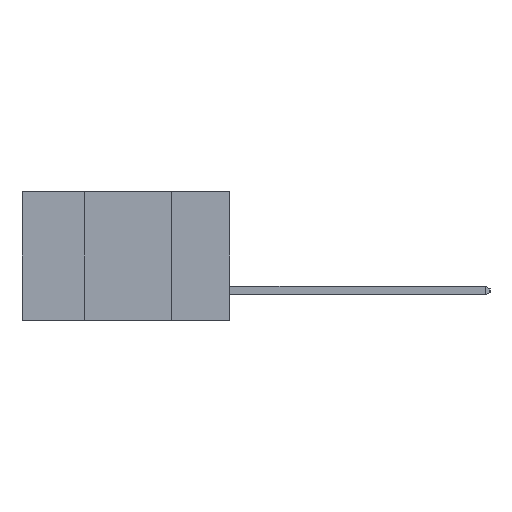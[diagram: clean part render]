
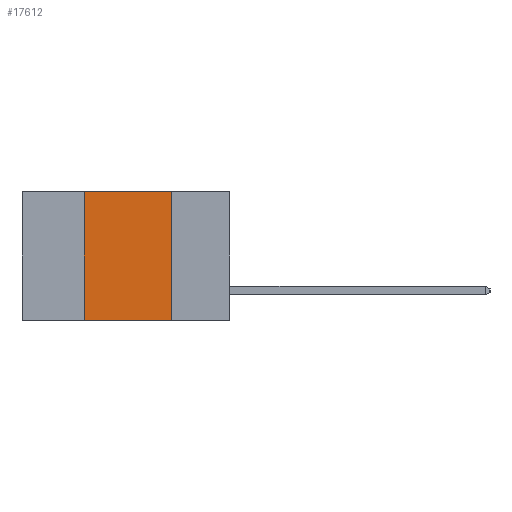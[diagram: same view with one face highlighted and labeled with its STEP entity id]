
A CAD part, left-side view. The second image highlights one B-rep face of the part: STEP entity #17612.
In plain terms, the highlighted planar face has unit normal (-1, 0, 0).
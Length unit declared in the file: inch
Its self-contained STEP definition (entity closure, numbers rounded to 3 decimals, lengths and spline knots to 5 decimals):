
#228 = ORIENTED_EDGE ( 'NONE', *, *, #11828, .T. ) ;
#694 = CARTESIAN_POINT ( 'NONE',  ( 0., 0.17, 0. ) ) ;
#741 = LINE ( 'NONE', #17571, #1330 ) ;
#1330 = VECTOR ( 'NONE', #17601, 39.37008 ) ;
#1515 = EDGE_LOOP ( 'NONE', ( #8583, #3149, #15815, #228 ) ) ;
#2476 = PLANE ( 'NONE',  #22331 ) ;
#3149 = ORIENTED_EDGE ( 'NONE', *, *, #5384, .F. ) ;
#4355 = DIRECTION ( 'NONE',  ( 1., 0., 0. ) ) ;
#4582 = VERTEX_POINT ( 'NONE', #12897 ) ;
#4764 = EDGE_CURVE ( 'NONE', #4582, #5262, #20066, .T. ) ;
#5262 = VERTEX_POINT ( 'NONE', #21990 ) ;
#5384 = EDGE_CURVE ( 'NONE', #5262, #23227, #741, .T. ) ;
#6442 = CARTESIAN_POINT ( 'NONE',  ( 0., 0.17, -0.37 ) ) ;
#8358 = LINE ( 'NONE', #22901, #22315 ) ;
#8583 = ORIENTED_EDGE ( 'NONE', *, *, #12006, .F. ) ;
#8634 = VECTOR ( 'NONE', #20306, 39.37008 ) ;
#8692 = CARTESIAN_POINT ( 'NONE',  ( 0., 0.42, -0.37 ) ) ;
#9062 = DIRECTION ( 'NONE',  ( 0., 0., 1. ) ) ;
#11828 = EDGE_CURVE ( 'NONE', #4582, #20578, #8358, .T. ) ;
#12006 = EDGE_CURVE ( 'NONE', #23227, #20578, #23127, .T. ) ;
#12897 = CARTESIAN_POINT ( 'NONE',  ( 0., 0.42, -0.37 ) ) ;
#13789 = FACE_OUTER_BOUND ( 'NONE', #1515, .T. ) ;
#15222 = VECTOR ( 'NONE', #9062, 39.37008 ) ;
#15347 = CARTESIAN_POINT ( 'NONE',  ( 0., 0.6, 0. ) ) ;
#15815 = ORIENTED_EDGE ( 'NONE', *, *, #4764, .F. ) ;
#17167 = DIRECTION ( 'NONE',  ( 0., 0., -1. ) ) ;
#17571 = CARTESIAN_POINT ( 'NONE',  ( 0., 0.6, 0. ) ) ;
#17601 = DIRECTION ( 'NONE',  ( 0., -1., 0. ) ) ;
#17612 = ADVANCED_FACE ( 'NONE', ( #13789 ), #2476, .F. ) ;
#20066 = LINE ( 'NONE', #8692, #15222 ) ;
#20306 = DIRECTION ( 'NONE',  ( 0., 0., -1. ) ) ;
#20331 = CARTESIAN_POINT ( 'NONE',  ( 0., 0.17, -0.37 ) ) ;
#20578 = VERTEX_POINT ( 'NONE', #6442 ) ;
#21990 = CARTESIAN_POINT ( 'NONE',  ( 0., 0.42, 0. ) ) ;
#22315 = VECTOR ( 'NONE', #23098, 39.37008 ) ;
#22331 = AXIS2_PLACEMENT_3D ( 'NONE', #15347, #4355, #17167 ) ;
#22901 = CARTESIAN_POINT ( 'NONE',  ( 0., 0.6, -0.37 ) ) ;
#23098 = DIRECTION ( 'NONE',  ( 0., -1., 0. ) ) ;
#23127 = LINE ( 'NONE', #20331, #8634 ) ;
#23227 = VERTEX_POINT ( 'NONE', #694 ) ;
